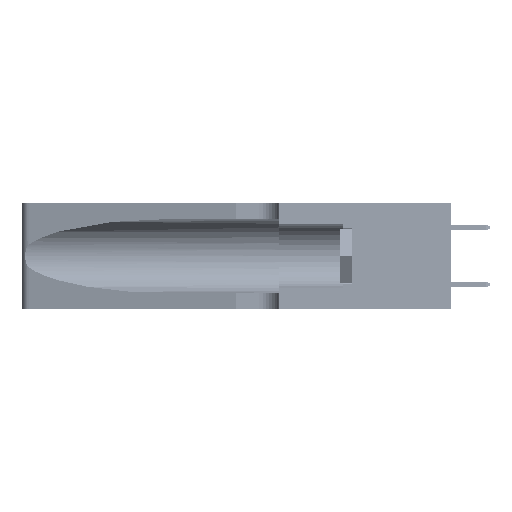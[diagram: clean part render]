
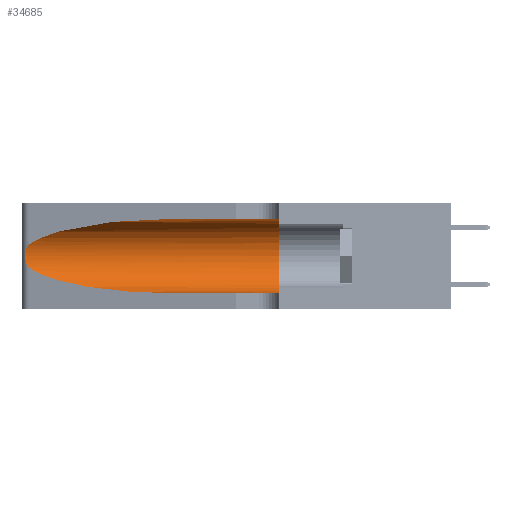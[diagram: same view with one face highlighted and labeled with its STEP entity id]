
A CAD part, left-side view. The second image highlights one B-rep face of the part: STEP entity #34685.
In plain terms, the highlighted cylindrical face has radius 3.308 mm (diameter 6.617 mm), a partial arc.
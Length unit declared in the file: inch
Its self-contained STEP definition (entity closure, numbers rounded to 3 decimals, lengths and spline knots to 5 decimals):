
#478 = ORIENTED_EDGE ( 'NONE', *, *, #14822, .F. ) ;
#1159 = DIRECTION ( 'NONE',  ( 0., -1., 0. ) ) ;
#3284 = DIRECTION ( 'NONE',  ( 0., -1., 0. ) ) ;
#3779 = CARTESIAN_POINT ( 'NONE',  ( 0.26075, 1.23896, 0.19203 ) ) ;
#7460 = DIRECTION ( 'NONE',  ( 0., 0., 1. ) ) ;
#7586 = CARTESIAN_POINT ( 'NONE',  ( 0.18966, 0.96281, 0.05475 ) ) ;
#7915 = CARTESIAN_POINT ( 'NONE',  ( 0.25856, 1.23593, 0.16098 ) ) ;
#8917 = FACE_OUTER_BOUND ( 'NONE', #14136, .T. ) ;
#9231 =( BOUNDED_CURVE ( )  B_SPLINE_CURVE ( 3, ( #29714, #16415, #7586, #28605 ),
 .UNSPECIFIED., .F., .T. ) 
 B_SPLINE_CURVE_WITH_KNOTS ( ( 4, 4 ),
 ( 3.44316, 4.71239 ),
 .UNSPECIFIED. ) 
 CURVE ( )  GEOMETRIC_REPRESENTATION_ITEM ( )  RATIONAL_B_SPLINE_CURVE ( ( 1., 0.87, 0.87, 1. ) ) 
 REPRESENTATION_ITEM ( '' )  );
#9802 = CARTESIAN_POINT ( 'NONE',  ( 0.1305, 0.72297, 0.31525 ) ) ;
#12147 = DIRECTION ( 'NONE',  ( 0., 1., 0. ) ) ;
#13160 = CIRCLE ( 'NONE', #20257, 0.13025 ) ;
#13363 = CARTESIAN_POINT ( 'NONE',  ( 0.1305, 1.61858, 0.185 ) ) ;
#13823 = VERTEX_POINT ( 'NONE', #14497 ) ;
#14136 = EDGE_LOOP ( 'NONE', ( #35881, #27996, #14665, #24463, #39812, #478 ) ) ;
#14497 = CARTESIAN_POINT ( 'NONE',  ( 0.25487, 1.22718, 0.14631 ) ) ;
#14665 = ORIENTED_EDGE ( 'NONE', *, *, #35890, .T. ) ;
#14822 = EDGE_CURVE ( 'NONE', #52813, #54448, #28169, .T. ) ;
#15925 = CARTESIAN_POINT ( 'NONE',  ( 0.25854, 1.2359, 0.20912 ) ) ;
#15997 = CARTESIAN_POINT ( 'NONE',  ( 0.18966, 0.96281, 0.31525 ) ) ;
#16415 = CARTESIAN_POINT ( 'NONE',  ( 0.2373, 1.15595, 0.08982 ) ) ;
#16749 = CARTESIAN_POINT ( 'NONE',  ( 0.25639, 1.23186, 0.15144 ) ) ;
#20257 = AXIS2_PLACEMENT_3D ( 'NONE', #50365, #12147, #7460 ) ;
#20591 = CARTESIAN_POINT ( 'NONE',  ( 0.1305, 0.35, 0.05475 ) ) ;
#20949 = CARTESIAN_POINT ( 'NONE',  ( 0.25639, 1.23184, 0.21858 ) ) ;
#24265 = CARTESIAN_POINT ( 'NONE',  ( 0.26017, 1.23833, 0.17102 ) ) ;
#24463 = ORIENTED_EDGE ( 'NONE', *, *, #40735, .T. ) ;
#25479 = CARTESIAN_POINT ( 'NONE',  ( 0.1305, 0.72297, 0.05475 ) ) ;
#25725 = B_SPLINE_CURVE_WITH_KNOTS ( 'NONE', 3,
 ( #37267, #53894, #20949, #45585, #15925, #37836, #3779, #29497, #24265, #7915, #48787, #16749, #33411, #28667 ),
 .UNSPECIFIED., .F., .F.,
 ( 4, 2, 2, 2, 2, 2, 4 ),
 ( 0., 0.00027, 0.00053, 0.00107, 0.0016, 0.00187, 0.00214 ),
 .UNSPECIFIED. ) ;
#27457 = DIRECTION ( 'NONE',  ( 0., -1., 0. ) ) ;
#27996 = ORIENTED_EDGE ( 'NONE', *, *, #50543, .T. ) ;
#28169 = LINE ( 'NONE', #41201, #45762 ) ;
#28605 = CARTESIAN_POINT ( 'NONE',  ( 0.1305, 0.72297, 0.05475 ) ) ;
#28667 = CARTESIAN_POINT ( 'NONE',  ( 0.25487, 1.22718, 0.14631 ) ) ;
#29497 = CARTESIAN_POINT ( 'NONE',  ( 0.26075, 1.23896, 0.178 ) ) ;
#29714 = CARTESIAN_POINT ( 'NONE',  ( 0.25487, 1.22718, 0.14631 ) ) ;
#30536 = CYLINDRICAL_SURFACE ( 'NONE', #48785, 0.13025 ) ;
#33411 = CARTESIAN_POINT ( 'NONE',  ( 0.25555, 1.22993, 0.14849 ) ) ;
#34044 = VERTEX_POINT ( 'NONE', #20591 ) ;
#34685 = ADVANCED_FACE ( 'NONE', ( #8917 ), #30536, .F. ) ;
#35121 = VECTOR ( 'NONE', #27457, 39.37008 ) ;
#35181 = VERTEX_POINT ( 'NONE', #25479 ) ;
#35466 = CARTESIAN_POINT ( 'NONE',  ( 0.1305, 0.72297, 0.31525 ) ) ;
#35881 = ORIENTED_EDGE ( 'NONE', *, *, #36710, .T. ) ;
#35890 = EDGE_CURVE ( 'NONE', #13823, #35181, #9231, .T. ) ;
#36710 = EDGE_CURVE ( 'NONE', #52813, #45926, #50310, .T. ) ;
#37267 = CARTESIAN_POINT ( 'NONE',  ( 0.25487, 1.22718, 0.22369 ) ) ;
#37836 = CARTESIAN_POINT ( 'NONE',  ( 0.26018, 1.23835, 0.19895 ) ) ;
#38053 = EDGE_CURVE ( 'NONE', #54448, #34044, #13160, .T. ) ;
#39812 = ORIENTED_EDGE ( 'NONE', *, *, #38053, .F. ) ;
#40735 = EDGE_CURVE ( 'NONE', #35181, #34044, #45460, .T. ) ;
#41201 = CARTESIAN_POINT ( 'NONE',  ( 0.1305, 1.61858, 0.31525 ) ) ;
#41509 = CARTESIAN_POINT ( 'NONE',  ( 0.25487, 1.22718, 0.22369 ) ) ;
#45460 = LINE ( 'NONE', #49351, #35121 ) ;
#45585 = CARTESIAN_POINT ( 'NONE',  ( 0.25787, 1.23484, 0.2124 ) ) ;
#45762 = VECTOR ( 'NONE', #3284, 39.37008 ) ;
#45926 = VERTEX_POINT ( 'NONE', #52012 ) ;
#46922 = DIRECTION ( 'NONE',  ( 0., 0., -1. ) ) ;
#48785 = AXIS2_PLACEMENT_3D ( 'NONE', #13363, #1159, #46922 ) ;
#48787 = CARTESIAN_POINT ( 'NONE',  ( 0.25789, 1.23486, 0.15765 ) ) ;
#49351 = CARTESIAN_POINT ( 'NONE',  ( 0.1305, 1.61858, 0.05475 ) ) ;
#50079 = CARTESIAN_POINT ( 'NONE',  ( 0.2373, 1.15595, 0.28018 ) ) ;
#50310 =( BOUNDED_CURVE ( )  B_SPLINE_CURVE ( 3, ( #35466, #15997, #50079, #41509 ),
 .UNSPECIFIED., .F., .F. ) 
 B_SPLINE_CURVE_WITH_KNOTS ( ( 4, 4 ),
 ( 1.5708, 2.84003 ),
 .UNSPECIFIED. ) 
 CURVE ( )  GEOMETRIC_REPRESENTATION_ITEM ( )  RATIONAL_B_SPLINE_CURVE ( ( 1., 0.87, 0.87, 1. ) ) 
 REPRESENTATION_ITEM ( '' )  );
#50365 = CARTESIAN_POINT ( 'NONE',  ( 0.1305, 0.35, 0.185 ) ) ;
#50543 = EDGE_CURVE ( 'NONE', #45926, #13823, #25725, .T. ) ;
#52012 = CARTESIAN_POINT ( 'NONE',  ( 0.25487, 1.22718, 0.22369 ) ) ;
#52813 = VERTEX_POINT ( 'NONE', #9802 ) ;
#53894 = CARTESIAN_POINT ( 'NONE',  ( 0.25555, 1.22994, 0.2215 ) ) ;
#54448 = VERTEX_POINT ( 'NONE', #54580 ) ;
#54580 = CARTESIAN_POINT ( 'NONE',  ( 0.1305, 0.35, 0.31525 ) ) ;
